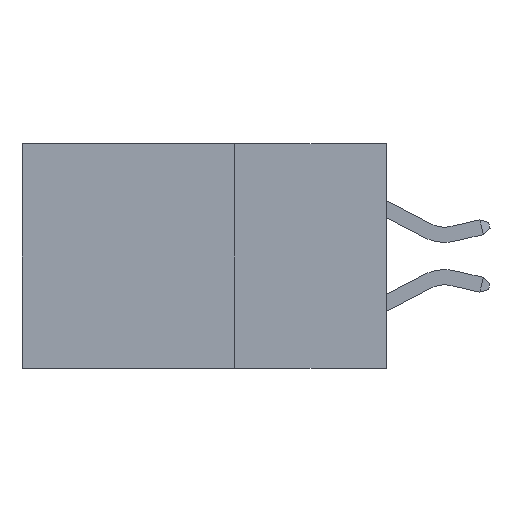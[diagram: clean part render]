
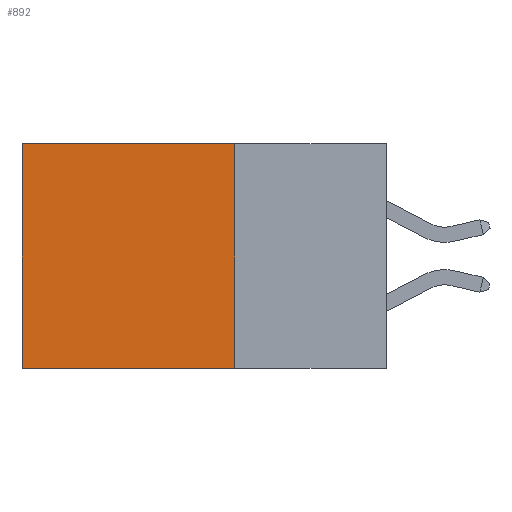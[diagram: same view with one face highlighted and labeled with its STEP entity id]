
A CAD part, left-side view. The second image highlights one B-rep face of the part: STEP entity #892.
In plain terms, the highlighted planar face has unit normal (-1, 0, 0).
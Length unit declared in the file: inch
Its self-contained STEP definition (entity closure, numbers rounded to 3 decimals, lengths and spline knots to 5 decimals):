
#15 = CARTESIAN_POINT ( 'NONE',  ( 0.2615, 0.25, 0. ) ) ;
#191 = DIRECTION ( 'NONE',  ( 0., 0., -1. ) ) ;
#278 = EDGE_CURVE ( 'NONE', #7450, #2281, #13468, .T. ) ;
#892 = ADVANCED_FACE ( 'NONE', ( #2735 ), #11708, .F. ) ;
#1061 = VECTOR ( 'NONE', #11823, 39.37008 ) ;
#1142 = ORIENTED_EDGE ( 'NONE', *, *, #2589, .T. ) ;
#1277 = CARTESIAN_POINT ( 'NONE',  ( 0.2615, 0.25, -0.37 ) ) ;
#1425 = CARTESIAN_POINT ( 'NONE',  ( 0.2615, 0.25, -0.37 ) ) ;
#1494 = CARTESIAN_POINT ( 'NONE',  ( 0.2615, 0.25, -0.37 ) ) ;
#1775 = DIRECTION ( 'NONE',  ( 1., 0., 0. ) ) ;
#2094 = VECTOR ( 'NONE', #12295, 39.37008 ) ;
#2281 = VERTEX_POINT ( 'NONE', #13095 ) ;
#2589 = EDGE_CURVE ( 'NONE', #13762, #2281, #7396, .T. ) ;
#2735 = FACE_OUTER_BOUND ( 'NONE', #13822, .T. ) ;
#4017 = EDGE_CURVE ( 'NONE', #4887, #13762, #10874, .T. ) ;
#4531 = ORIENTED_EDGE ( 'NONE', *, *, #7455, .F. ) ;
#4887 = VERTEX_POINT ( 'NONE', #7159 ) ;
#5762 = LINE ( 'NONE', #1277, #9744 ) ;
#7159 = CARTESIAN_POINT ( 'NONE',  ( 0.2615, 0.25, 0. ) ) ;
#7396 = LINE ( 'NONE', #12795, #1061 ) ;
#7450 = VERTEX_POINT ( 'NONE', #1425 ) ;
#7455 = EDGE_CURVE ( 'NONE', #4887, #7450, #5762, .T. ) ;
#7836 = CARTESIAN_POINT ( 'NONE',  ( 0.2615, 0.6, 0. ) ) ;
#9425 = AXIS2_PLACEMENT_3D ( 'NONE', #1494, #1775, #11638 ) ;
#9744 = VECTOR ( 'NONE', #191, 39.37008 ) ;
#9995 = VECTOR ( 'NONE', #11983, 39.37008 ) ;
#10674 = ORIENTED_EDGE ( 'NONE', *, *, #4017, .T. ) ;
#10874 = LINE ( 'NONE', #15, #9995 ) ;
#11638 = DIRECTION ( 'NONE',  ( 0., 0., -1. ) ) ;
#11708 = PLANE ( 'NONE',  #9425 ) ;
#11823 = DIRECTION ( 'NONE',  ( 0., 0., -1. ) ) ;
#11983 = DIRECTION ( 'NONE',  ( 0., 1., 0. ) ) ;
#12258 = ORIENTED_EDGE ( 'NONE', *, *, #278, .F. ) ;
#12295 = DIRECTION ( 'NONE',  ( 0., 1., 0. ) ) ;
#12795 = CARTESIAN_POINT ( 'NONE',  ( 0.2615, 0.6, -0.37 ) ) ;
#13095 = CARTESIAN_POINT ( 'NONE',  ( 0.2615, 0.6, -0.37 ) ) ;
#13397 = CARTESIAN_POINT ( 'NONE',  ( 0.2615, 0.25, -0.37 ) ) ;
#13468 = LINE ( 'NONE', #13397, #2094 ) ;
#13762 = VERTEX_POINT ( 'NONE', #7836 ) ;
#13822 = EDGE_LOOP ( 'NONE', ( #1142, #12258, #4531, #10674 ) ) ;
